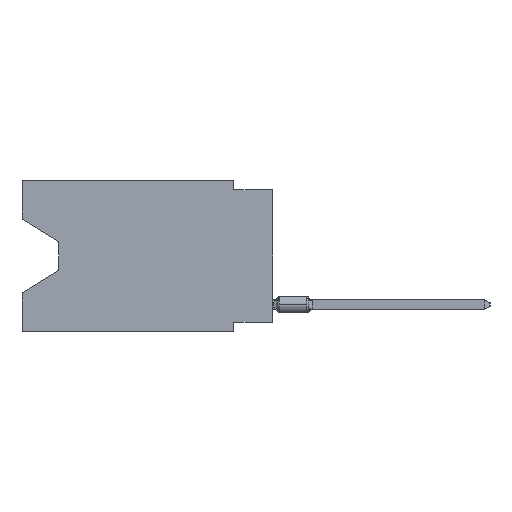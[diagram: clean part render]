
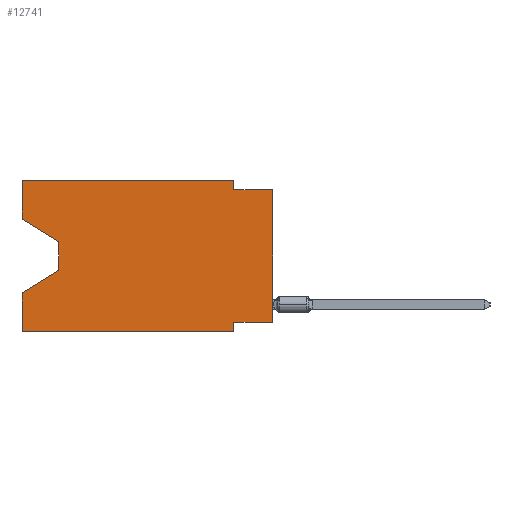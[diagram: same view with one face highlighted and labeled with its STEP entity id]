
A CAD part, left-side view. The second image highlights one B-rep face of the part: STEP entity #12741.
In plain terms, the highlighted planar face has unit normal (-1, 0, 0).
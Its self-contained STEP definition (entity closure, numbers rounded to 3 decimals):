
#641 = DIRECTION ( 'NONE',  ( 0., 0., 1. ) ) ;
#1213 = CARTESIAN_POINT ( 'NONE',  ( 0., 16.383, -2.546 ) ) ;
#1817 = LINE ( 'NONE', #56778, #8698 ) ;
#2169 = VERTEX_POINT ( 'NONE', #2898 ) ;
#2898 = CARTESIAN_POINT ( 'NONE',  ( 0., 13.97, -5.893 ) ) ;
#3500 = DIRECTION ( 'NONE',  ( 0., -1., 0. ) ) ;
#5035 = LINE ( 'NONE', #66435, #28671 ) ;
#7752 = ORIENTED_EDGE ( 'NONE', *, *, #9857, .F. ) ;
#8698 = VECTOR ( 'NONE', #26059, 1000. ) ;
#9857 = EDGE_CURVE ( 'NONE', #24155, #65973, #50494, .T. ) ;
#11284 = CARTESIAN_POINT ( 'NONE',  ( 0., 16.383, 0. ) ) ;
#12467 = VECTOR ( 'NONE', #66838, 1000. ) ;
#12741 = ADVANCED_FACE ( 'NONE', ( #19148 ), #42219, .F. ) ;
#15554 = CARTESIAN_POINT ( 'NONE',  ( 0., 0., -9.271 ) ) ;
#17001 = EDGE_LOOP ( 'NONE', ( #54631, #46494, #39755, #43298, #17402, #72571, #31196, #35246, #64129, #74858, #68146, #7752 ) ) ;
#17402 = ORIENTED_EDGE ( 'NONE', *, *, #65446, .T. ) ;
#18226 = LINE ( 'NONE', #61473, #45819 ) ;
#18360 = DIRECTION ( 'NONE',  ( 1., 0., 0. ) ) ;
#19148 = FACE_OUTER_BOUND ( 'NONE', #17001, .T. ) ;
#20164 = DIRECTION ( 'NONE',  ( 0., 0., 1. ) ) ;
#20685 = DIRECTION ( 'NONE',  ( 0., -1., 0. ) ) ;
#22072 = CARTESIAN_POINT ( 'NONE',  ( 0., 16.383, 0. ) ) ;
#23326 = VECTOR ( 'NONE', #20685, 1000. ) ;
#23394 = LINE ( 'NONE', #71206, #23326 ) ;
#23725 = CARTESIAN_POINT ( 'NONE',  ( 0., 2.54, 0. ) ) ;
#24155 = VERTEX_POINT ( 'NONE', #64271 ) ;
#24931 = CARTESIAN_POINT ( 'NONE',  ( 0., 13.97, -4.013 ) ) ;
#25183 = DIRECTION ( 'NONE',  ( 0., 0.855, -0.519 ) ) ;
#25312 = VECTOR ( 'NONE', #25183, 1000. ) ;
#25857 = DIRECTION ( 'NONE',  ( 0., -0.855, -0.519 ) ) ;
#25950 = CARTESIAN_POINT ( 'NONE',  ( 0., 2.54, 0. ) ) ;
#26059 = DIRECTION ( 'NONE',  ( 0., -1., 0. ) ) ;
#27050 = EDGE_CURVE ( 'NONE', #27393, #76769, #42291, .T. ) ;
#27393 = VERTEX_POINT ( 'NONE', #15554 ) ;
#27764 = LINE ( 'NONE', #60795, #12467 ) ;
#28138 = VECTOR ( 'NONE', #57483, 1000. ) ;
#28671 = VECTOR ( 'NONE', #72921, 1000. ) ;
#30718 = CARTESIAN_POINT ( 'NONE',  ( 0., 16.383, 0. ) ) ;
#31196 = ORIENTED_EDGE ( 'NONE', *, *, #60866, .F. ) ;
#31544 = VERTEX_POINT ( 'NONE', #74912 ) ;
#35246 = ORIENTED_EDGE ( 'NONE', *, *, #27050, .T. ) ;
#35866 = EDGE_CURVE ( 'NONE', #52238, #67664, #27764, .T. ) ;
#35992 = EDGE_CURVE ( 'NONE', #2169, #67664, #61974, .T. ) ;
#36782 = LINE ( 'NONE', #1213, #78393 ) ;
#37367 = CARTESIAN_POINT ( 'NONE',  ( 0., 16.383, -7.36 ) ) ;
#37703 = LINE ( 'NONE', #56298, #28138 ) ;
#39755 = ORIENTED_EDGE ( 'NONE', *, *, #35992, .T. ) ;
#41197 = VECTOR ( 'NONE', #3500, 1000. ) ;
#41940 = VERTEX_POINT ( 'NONE', #44496 ) ;
#42219 = PLANE ( 'NONE',  #52845 ) ;
#42291 = LINE ( 'NONE', #43479, #61264 ) ;
#42534 = VERTEX_POINT ( 'NONE', #23725 ) ;
#43298 = ORIENTED_EDGE ( 'NONE', *, *, #35866, .F. ) ;
#43479 = CARTESIAN_POINT ( 'NONE',  ( 0., 0., 0. ) ) ;
#44180 = CARTESIAN_POINT ( 'NONE',  ( 0., 13.97, -5.893 ) ) ;
#44496 = CARTESIAN_POINT ( 'NONE',  ( 0., 2.54, -0.635 ) ) ;
#45819 = VECTOR ( 'NONE', #55010, 1000. ) ;
#46494 = ORIENTED_EDGE ( 'NONE', *, *, #77916, .T. ) ;
#47072 = VERTEX_POINT ( 'NONE', #24931 ) ;
#49149 = EDGE_CURVE ( 'NONE', #42534, #41940, #57064, .T. ) ;
#49202 = CARTESIAN_POINT ( 'NONE',  ( 0., 2.54, -9.906 ) ) ;
#50020 = EDGE_CURVE ( 'NONE', #31544, #72736, #5035, .T. ) ;
#50494 = LINE ( 'NONE', #30718, #69229 ) ;
#52238 = VERTEX_POINT ( 'NONE', #76324 ) ;
#52790 = LINE ( 'NONE', #22072, #41197 ) ;
#52845 = AXIS2_PLACEMENT_3D ( 'NONE', #73741, #18360, #66870 ) ;
#54631 = ORIENTED_EDGE ( 'NONE', *, *, #57977, .T. ) ;
#55010 = DIRECTION ( 'NONE',  ( 0., 0., -1. ) ) ;
#56298 = CARTESIAN_POINT ( 'NONE',  ( 0., 0., -9.271 ) ) ;
#56778 = CARTESIAN_POINT ( 'NONE',  ( 0., 16.383, -9.906 ) ) ;
#57064 = LINE ( 'NONE', #25950, #64733 ) ;
#57483 = DIRECTION ( 'NONE',  ( 0., 1., 0. ) ) ;
#57977 = EDGE_CURVE ( 'NONE', #24155, #47072, #36782, .T. ) ;
#58875 = EDGE_CURVE ( 'NONE', #65973, #42534, #52790, .T. ) ;
#60795 = CARTESIAN_POINT ( 'NONE',  ( 0., 16.383, 0. ) ) ;
#60866 = EDGE_CURVE ( 'NONE', #27393, #31544, #37703, .T. ) ;
#61264 = VECTOR ( 'NONE', #641, 1000. ) ;
#61473 = CARTESIAN_POINT ( 'NONE',  ( 0., 13.97, -4.013 ) ) ;
#61974 = LINE ( 'NONE', #44180, #25312 ) ;
#63524 = DIRECTION ( 'NONE',  ( 0., 0., -1. ) ) ;
#64129 = ORIENTED_EDGE ( 'NONE', *, *, #65983, .F. ) ;
#64271 = CARTESIAN_POINT ( 'NONE',  ( 0., 16.383, -2.546 ) ) ;
#64733 = VECTOR ( 'NONE', #63524, 1000. ) ;
#65446 = EDGE_CURVE ( 'NONE', #52238, #72736, #1817, .T. ) ;
#65973 = VERTEX_POINT ( 'NONE', #11284 ) ;
#65983 = EDGE_CURVE ( 'NONE', #41940, #76769, #23394, .T. ) ;
#66435 = CARTESIAN_POINT ( 'NONE',  ( 0., 2.54, -9.906 ) ) ;
#66838 = DIRECTION ( 'NONE',  ( 0., 0., 1. ) ) ;
#66870 = DIRECTION ( 'NONE',  ( 0., 0., -1. ) ) ;
#67664 = VERTEX_POINT ( 'NONE', #37367 ) ;
#68146 = ORIENTED_EDGE ( 'NONE', *, *, #58875, .F. ) ;
#68310 = CARTESIAN_POINT ( 'NONE',  ( 0., 0., -0.635 ) ) ;
#69229 = VECTOR ( 'NONE', #20164, 1000. ) ;
#71206 = CARTESIAN_POINT ( 'NONE',  ( 0., 0., -0.635 ) ) ;
#72571 = ORIENTED_EDGE ( 'NONE', *, *, #50020, .F. ) ;
#72736 = VERTEX_POINT ( 'NONE', #49202 ) ;
#72921 = DIRECTION ( 'NONE',  ( 0., 0., -1. ) ) ;
#73741 = CARTESIAN_POINT ( 'NONE',  ( 0., 16.383, 0. ) ) ;
#74858 = ORIENTED_EDGE ( 'NONE', *, *, #49149, .F. ) ;
#74912 = CARTESIAN_POINT ( 'NONE',  ( 0., 2.54, -9.271 ) ) ;
#76324 = CARTESIAN_POINT ( 'NONE',  ( 0., 16.383, -9.906 ) ) ;
#76769 = VERTEX_POINT ( 'NONE', #68310 ) ;
#77916 = EDGE_CURVE ( 'NONE', #47072, #2169, #18226, .T. ) ;
#78393 = VECTOR ( 'NONE', #25857, 1000. ) ;
